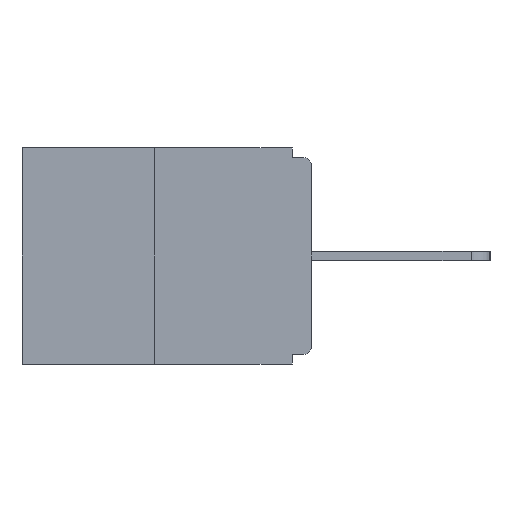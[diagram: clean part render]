
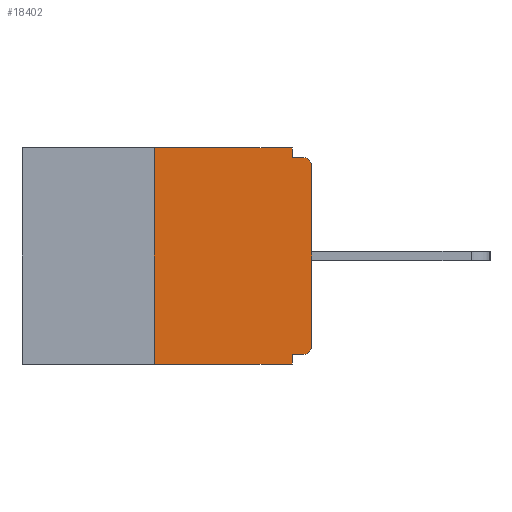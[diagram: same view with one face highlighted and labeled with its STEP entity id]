
A CAD part, left-side view. The second image highlights one B-rep face of the part: STEP entity #18402.
In plain terms, the highlighted planar face has unit normal (-1, 0, 0).
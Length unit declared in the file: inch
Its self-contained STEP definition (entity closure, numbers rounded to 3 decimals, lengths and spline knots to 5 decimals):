
#86 = CARTESIAN_POINT ( 'NONE',  ( 0., 0.031, -0.343 ) ) ;
#384 = DIRECTION ( 'NONE',  ( 0., 0., 1. ) ) ;
#423 = VERTEX_POINT ( 'NONE', #14056 ) ;
#525 = CARTESIAN_POINT ( 'NONE',  ( 0., 0., -0.313 ) ) ;
#847 = VECTOR ( 'NONE', #2214, 39.37008 ) ;
#897 = ORIENTED_EDGE ( 'NONE', *, *, #11152, .T. ) ;
#1345 = CARTESIAN_POINT ( 'NONE',  ( 0., 0.46, -0.343 ) ) ;
#1386 = AXIS2_PLACEMENT_3D ( 'NONE', #20357, #9083, #20120 ) ;
#1669 = VECTOR ( 'NONE', #5172, 39.37008 ) ;
#1965 = CARTESIAN_POINT ( 'NONE',  ( 0., 0.46, 0. ) ) ;
#2214 = DIRECTION ( 'NONE',  ( 0., 0., -1. ) ) ;
#2442 = LINE ( 'NONE', #20441, #847 ) ;
#2482 = VERTEX_POINT ( 'NONE', #15925 ) ;
#3374 = ORIENTED_EDGE ( 'NONE', *, *, #18299, .F. ) ;
#3970 = CARTESIAN_POINT ( 'NONE',  ( 0., 0., 0. ) ) ;
#3997 = FACE_OUTER_BOUND ( 'NONE', #20717, .T. ) ;
#4400 = LINE ( 'NONE', #9690, #7514 ) ;
#5172 = DIRECTION ( 'NONE',  ( 0., -1., 0. ) ) ;
#5566 = AXIS2_PLACEMENT_3D ( 'NONE', #14753, #16919, #20046 ) ;
#5692 = DIRECTION ( 'NONE',  ( 0., -1., 0. ) ) ;
#5699 = VECTOR ( 'NONE', #9283, 39.37008 ) ;
#5791 = PLANE ( 'NONE',  #8267 ) ;
#5989 = CARTESIAN_POINT ( 'NONE',  ( 0., 0.015, -0.328 ) ) ;
#7305 = EDGE_CURVE ( 'NONE', #7901, #20939, #18411, .T. ) ;
#7463 = LINE ( 'NONE', #3970, #19580 ) ;
#7497 = ORIENTED_EDGE ( 'NONE', *, *, #19913, .F. ) ;
#7498 = CARTESIAN_POINT ( 'NONE',  ( 0., 0., -0.328 ) ) ;
#7514 = VECTOR ( 'NONE', #7888, 39.37008 ) ;
#7888 = DIRECTION ( 'NONE',  ( 0., 0., 1. ) ) ;
#7901 = VERTEX_POINT ( 'NONE', #21691 ) ;
#8267 = AXIS2_PLACEMENT_3D ( 'NONE', #16625, #19008, #9534 ) ;
#9083 = DIRECTION ( 'NONE',  ( -1., 0., 0. ) ) ;
#9283 = DIRECTION ( 'NONE',  ( 0., -1., 0. ) ) ;
#9534 = DIRECTION ( 'NONE',  ( 0., 0., -1. ) ) ;
#9690 = CARTESIAN_POINT ( 'NONE',  ( 0., 0.25, 0. ) ) ;
#10140 = VERTEX_POINT ( 'NONE', #5989 ) ;
#10791 = EDGE_CURVE ( 'NONE', #2482, #19240, #23666, .T. ) ;
#10827 = VERTEX_POINT ( 'NONE', #86 ) ;
#10888 = DIRECTION ( 'NONE',  ( 0., 1., 0. ) ) ;
#11152 = EDGE_CURVE ( 'NONE', #423, #10827, #15872, .T. ) ;
#11415 = ORIENTED_EDGE ( 'NONE', *, *, #22925, .T. ) ;
#11876 = EDGE_CURVE ( 'NONE', #423, #7901, #4400, .T. ) ;
#13339 = VECTOR ( 'NONE', #10888, 39.37008 ) ;
#13588 = CARTESIAN_POINT ( 'NONE',  ( 0., 0.031, -0.328 ) ) ;
#14056 = CARTESIAN_POINT ( 'NONE',  ( 0., 0.25, -0.343 ) ) ;
#14372 = CARTESIAN_POINT ( 'NONE',  ( 0., 0., -0.015 ) ) ;
#14392 = ORIENTED_EDGE ( 'NONE', *, *, #18067, .T. ) ;
#14753 = CARTESIAN_POINT ( 'NONE',  ( 0., 0.015, -0.03 ) ) ;
#14761 = CARTESIAN_POINT ( 'NONE',  ( 0., 0.015, -0.015 ) ) ;
#14773 = CIRCLE ( 'NONE', #5566, 0.015 ) ;
#15477 = EDGE_CURVE ( 'NONE', #17399, #10827, #2442, .T. ) ;
#15872 = LINE ( 'NONE', #1345, #1669 ) ;
#15925 = CARTESIAN_POINT ( 'NONE',  ( 0., 0.031, -0.015 ) ) ;
#16358 = ORIENTED_EDGE ( 'NONE', *, *, #17224, .T. ) ;
#16405 = VERTEX_POINT ( 'NONE', #17740 ) ;
#16625 = CARTESIAN_POINT ( 'NONE',  ( 0., 0.46, 0. ) ) ;
#16745 = VECTOR ( 'NONE', #5692, 39.37008 ) ;
#16807 = VERTEX_POINT ( 'NONE', #525 ) ;
#16919 = DIRECTION ( 'NONE',  ( -1., 0., 0. ) ) ;
#17224 = EDGE_CURVE ( 'NONE', #16807, #16405, #7463, .T. ) ;
#17399 = VERTEX_POINT ( 'NONE', #13588 ) ;
#17740 = CARTESIAN_POINT ( 'NONE',  ( 0., 0., -0.03 ) ) ;
#18067 = EDGE_CURVE ( 'NONE', #16405, #19240, #14773, .T. ) ;
#18299 = EDGE_CURVE ( 'NONE', #20939, #2482, #19667, .T. ) ;
#18402 = ADVANCED_FACE ( 'NONE', ( #3997 ), #5791, .F. ) ;
#18411 = LINE ( 'NONE', #1965, #5699 ) ;
#19006 = CIRCLE ( 'NONE', #1386, 0.015 ) ;
#19008 = DIRECTION ( 'NONE',  ( 1., 0., 0. ) ) ;
#19240 = VERTEX_POINT ( 'NONE', #14761 ) ;
#19388 = VECTOR ( 'NONE', #21326, 39.37008 ) ;
#19580 = VECTOR ( 'NONE', #384, 39.37008 ) ;
#19648 = ORIENTED_EDGE ( 'NONE', *, *, #11876, .F. ) ;
#19667 = LINE ( 'NONE', #23113, #19388 ) ;
#19824 = ORIENTED_EDGE ( 'NONE', *, *, #15477, .F. ) ;
#19913 = EDGE_CURVE ( 'NONE', #10140, #17399, #23548, .T. ) ;
#20046 = DIRECTION ( 'NONE',  ( 0., 0., -1. ) ) ;
#20120 = DIRECTION ( 'NONE',  ( 0., 0., -1. ) ) ;
#20357 = CARTESIAN_POINT ( 'NONE',  ( 0., 0.015, -0.313 ) ) ;
#20441 = CARTESIAN_POINT ( 'NONE',  ( 0., 0.031, -0.343 ) ) ;
#20717 = EDGE_LOOP ( 'NONE', ( #23593, #19648, #897, #19824, #7497, #11415, #16358, #14392, #23482, #3374 ) ) ;
#20839 = CARTESIAN_POINT ( 'NONE',  ( 0., 0.031, 0. ) ) ;
#20939 = VERTEX_POINT ( 'NONE', #20839 ) ;
#21326 = DIRECTION ( 'NONE',  ( 0., 0., -1. ) ) ;
#21691 = CARTESIAN_POINT ( 'NONE',  ( 0., 0.25, 0. ) ) ;
#22925 = EDGE_CURVE ( 'NONE', #10140, #16807, #19006, .T. ) ;
#23113 = CARTESIAN_POINT ( 'NONE',  ( 0., 0.031, 0. ) ) ;
#23482 = ORIENTED_EDGE ( 'NONE', *, *, #10791, .F. ) ;
#23548 = LINE ( 'NONE', #7498, #13339 ) ;
#23593 = ORIENTED_EDGE ( 'NONE', *, *, #7305, .F. ) ;
#23666 = LINE ( 'NONE', #14372, #16745 ) ;
